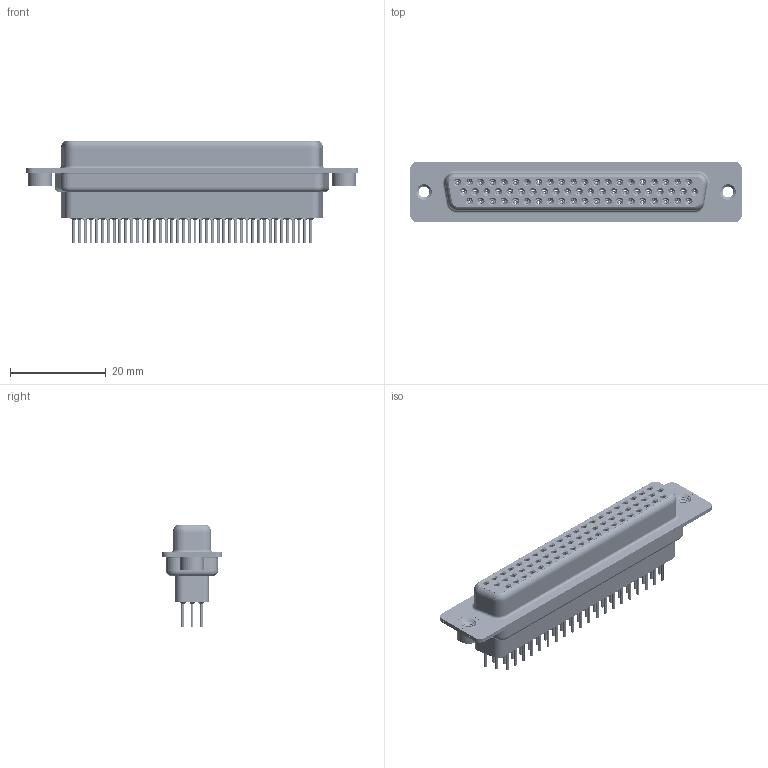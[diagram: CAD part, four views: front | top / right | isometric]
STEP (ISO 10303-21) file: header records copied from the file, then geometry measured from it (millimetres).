
FILE_DESCRIPTION (( 'STEP AP203' ), '1' );
FILE_NAME ('638-062-231-252.STEP', '2020-07-19T01:05:58', ( '' ), ( '' ), 'SwSTEP 2.0', 'SolidWorks 2020', '' );
FILE_SCHEMA (( 'CONFIG_CONTROL_DESIGN' ));
Length unit declared in the file: millimetre
Products named in the file (8): 638 4-40 Threaded Rivet; 638-062-231-252; 638 Housing_62 Contacts HP; 638 Shell Rear_62 Contacts; 638 Contact Row 1_31; 638 Shell Front_62 Contacts; 638 Contact Row 2_31; 638 Contact Row 3_31
Assembly tree (67 placements, depth 2):
  638-062-231-252
    638 Housing_62 Contacts HP
    638 Shell Front_62 Contacts
    638 Shell Rear_62 Contacts
    638 Contact Row 1_31  x21
    638 Contact Row 2_31  x21
    638 Contact Row 3_31  x20
    638 4-40 Threaded Rivet  x2
Bounding box: 69.32 x 12.6 x 21.5 mm (x, y, z)
Volume: 5643.2 mm3; surface area: 21118 mm2
Topology: 67 solids, 67 shells, 7905 faces, 20277 edges, 12641 vertices
Faces by surface type: cylinder 2183, plane 1989, torus 1545, bspline 1246, cone 942
Entity records: 46885 total; most frequent: CARTESIAN_POINT 11889, DIRECTION 7318, ORIENTED_EDGE 6402, EDGE_CURVE 3201, AXIS2_PLACEMENT_3D 3096, VERTEX_POINT 2028, EDGE_LOOP 1715, CIRCLE 1707
